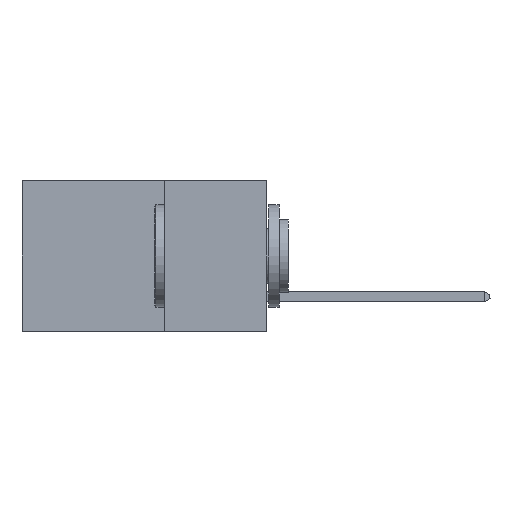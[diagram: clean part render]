
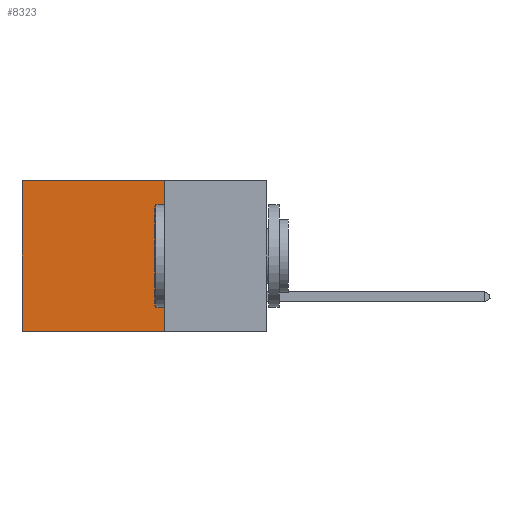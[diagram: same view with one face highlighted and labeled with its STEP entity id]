
A CAD part, left-side view. The second image highlights one B-rep face of the part: STEP entity #8323.
In plain terms, the highlighted planar face has unit normal (-1, 0, 0).
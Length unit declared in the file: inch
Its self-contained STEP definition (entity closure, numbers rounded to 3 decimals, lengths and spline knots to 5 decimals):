
#263 = CARTESIAN_POINT ( 'NONE',  ( 0.2875, 0.25, 0. ) ) ;
#318 = LINE ( 'NONE', #263, #18591 ) ;
#970 = ORIENTED_EDGE ( 'NONE', *, *, #5118, .T. ) ;
#1114 = LINE ( 'NONE', #8717, #16061 ) ;
#1580 = DIRECTION ( 'NONE',  ( 0., 1., 0. ) ) ;
#2949 = VERTEX_POINT ( 'NONE', #12368 ) ;
#3354 = EDGE_CURVE ( 'NONE', #9580, #11401, #6499, .T. ) ;
#3598 = CARTESIAN_POINT ( 'NONE',  ( 0.2875, 0.25, -0.37 ) ) ;
#3638 = ORIENTED_EDGE ( 'NONE', *, *, #7667, .T. ) ;
#5118 = EDGE_CURVE ( 'NONE', #2949, #14236, #1114, .T. ) ;
#5154 = ORIENTED_EDGE ( 'NONE', *, *, #11287, .F. ) ;
#5558 = VECTOR ( 'NONE', #1580, 39.37008 ) ;
#6499 = LINE ( 'NONE', #13287, #5558 ) ;
#6751 = LINE ( 'NONE', #16929, #10184 ) ;
#7477 = EDGE_LOOP ( 'NONE', ( #3638, #8996, #5154, #970 ) ) ;
#7667 = EDGE_CURVE ( 'NONE', #14236, #11401, #6751, .T. ) ;
#8323 = ADVANCED_FACE ( 'NONE', ( #11272 ), #14383, .F. ) ;
#8686 = DIRECTION ( 'NONE',  ( 1., 0., 0. ) ) ;
#8717 = CARTESIAN_POINT ( 'NONE',  ( 0.2875, 0.25, 0. ) ) ;
#8996 = ORIENTED_EDGE ( 'NONE', *, *, #3354, .F. ) ;
#9065 = DIRECTION ( 'NONE',  ( 0., 0., -1. ) ) ;
#9580 = VERTEX_POINT ( 'NONE', #3598 ) ;
#9849 = DIRECTION ( 'NONE',  ( 0., 0., -1. ) ) ;
#10184 = VECTOR ( 'NONE', #9849, 39.37008 ) ;
#11272 = FACE_OUTER_BOUND ( 'NONE', #7477, .T. ) ;
#11287 = EDGE_CURVE ( 'NONE', #2949, #9580, #318, .T. ) ;
#11401 = VERTEX_POINT ( 'NONE', #16405 ) ;
#12368 = CARTESIAN_POINT ( 'NONE',  ( 0.2875, 0.25, 0. ) ) ;
#13287 = CARTESIAN_POINT ( 'NONE',  ( 0.2875, 0.25, -0.37 ) ) ;
#14236 = VERTEX_POINT ( 'NONE', #17267 ) ;
#14383 = PLANE ( 'NONE',  #17564 ) ;
#16061 = VECTOR ( 'NONE', #17317, 39.37008 ) ;
#16405 = CARTESIAN_POINT ( 'NONE',  ( 0.2875, 0.6, -0.37 ) ) ;
#16929 = CARTESIAN_POINT ( 'NONE',  ( 0.2875, 0.6, 0. ) ) ;
#17229 = CARTESIAN_POINT ( 'NONE',  ( 0.2875, 0.25, 0. ) ) ;
#17267 = CARTESIAN_POINT ( 'NONE',  ( 0.2875, 0.6, 0. ) ) ;
#17317 = DIRECTION ( 'NONE',  ( 0., 1., 0. ) ) ;
#17564 = AXIS2_PLACEMENT_3D ( 'NONE', #17229, #8686, #18616 ) ;
#18591 = VECTOR ( 'NONE', #9065, 39.37008 ) ;
#18616 = DIRECTION ( 'NONE',  ( 0., 0., -1. ) ) ;
